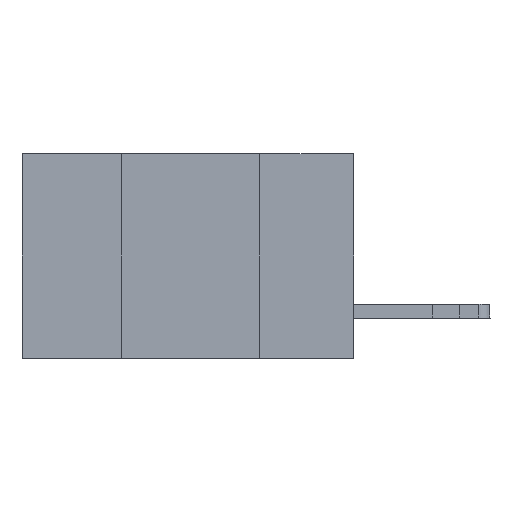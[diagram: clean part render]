
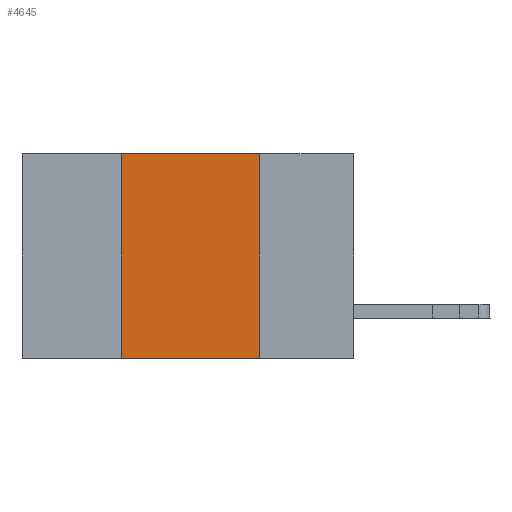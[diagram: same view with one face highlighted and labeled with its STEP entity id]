
A CAD part, left-side view. The second image highlights one B-rep face of the part: STEP entity #4645.
In plain terms, the highlighted planar face has unit normal (-1, 0, 0).
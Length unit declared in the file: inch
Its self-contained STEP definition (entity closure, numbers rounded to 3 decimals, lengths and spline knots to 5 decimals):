
#528 = DIRECTION ( 'NONE',  ( 0., 0., -1. ) ) ;
#1785 = EDGE_CURVE ( 'NONE', #28203, #6008, #26734, .T. ) ;
#3013 = CARTESIAN_POINT ( 'NONE',  ( 0., 0.6, 0. ) ) ;
#3293 = CARTESIAN_POINT ( 'NONE',  ( 0., 0.42, 0. ) ) ;
#3377 = ORIENTED_EDGE ( 'NONE', *, *, #24448, .F. ) ;
#4613 = CARTESIAN_POINT ( 'NONE',  ( 0., 0.42, -0.37 ) ) ;
#4645 = ADVANCED_FACE ( 'NONE', ( #11287 ), #28024, .F. ) ;
#4876 = CARTESIAN_POINT ( 'NONE',  ( 0., 0.17, -0.37 ) ) ;
#4970 = EDGE_CURVE ( 'NONE', #28203, #10147, #19681, .T. ) ;
#5333 = CARTESIAN_POINT ( 'NONE',  ( 0., 0.17, 0. ) ) ;
#6008 = VERTEX_POINT ( 'NONE', #4876 ) ;
#6701 = ORIENTED_EDGE ( 'NONE', *, *, #4970, .F. ) ;
#8340 = ORIENTED_EDGE ( 'NONE', *, *, #27097, .F. ) ;
#8568 = CARTESIAN_POINT ( 'NONE',  ( 0., 0.17, 0. ) ) ;
#10147 = VERTEX_POINT ( 'NONE', #12953 ) ;
#10848 = EDGE_LOOP ( 'NONE', ( #3377, #8340, #6701, #26213 ) ) ;
#11103 = VECTOR ( 'NONE', #528, 39.37008 ) ;
#11287 = FACE_OUTER_BOUND ( 'NONE', #10848, .T. ) ;
#12953 = CARTESIAN_POINT ( 'NONE',  ( 0., 0.42, 0. ) ) ;
#13492 = VECTOR ( 'NONE', #24445, 39.37008 ) ;
#15951 = AXIS2_PLACEMENT_3D ( 'NONE', #30255, #30352, #16408 ) ;
#16408 = DIRECTION ( 'NONE',  ( 0., 0., -1. ) ) ;
#19486 = DIRECTION ( 'NONE',  ( 0., -1., 0. ) ) ;
#19681 = LINE ( 'NONE', #3293, #13492 ) ;
#20528 = VECTOR ( 'NONE', #20784, 39.37008 ) ;
#20784 = DIRECTION ( 'NONE',  ( 0., -1., 0. ) ) ;
#21336 = CARTESIAN_POINT ( 'NONE',  ( 0., 0.6, -0.37 ) ) ;
#23991 = VERTEX_POINT ( 'NONE', #8568 ) ;
#24203 = LINE ( 'NONE', #3013, #24925 ) ;
#24445 = DIRECTION ( 'NONE',  ( 0., 0., 1. ) ) ;
#24448 = EDGE_CURVE ( 'NONE', #23991, #6008, #29734, .T. ) ;
#24925 = VECTOR ( 'NONE', #19486, 39.37008 ) ;
#26213 = ORIENTED_EDGE ( 'NONE', *, *, #1785, .T. ) ;
#26734 = LINE ( 'NONE', #21336, #20528 ) ;
#27097 = EDGE_CURVE ( 'NONE', #10147, #23991, #24203, .T. ) ;
#28024 = PLANE ( 'NONE',  #15951 ) ;
#28203 = VERTEX_POINT ( 'NONE', #4613 ) ;
#29734 = LINE ( 'NONE', #5333, #11103 ) ;
#30255 = CARTESIAN_POINT ( 'NONE',  ( 0., 0.6, 0. ) ) ;
#30352 = DIRECTION ( 'NONE',  ( 1., 0., 0. ) ) ;
